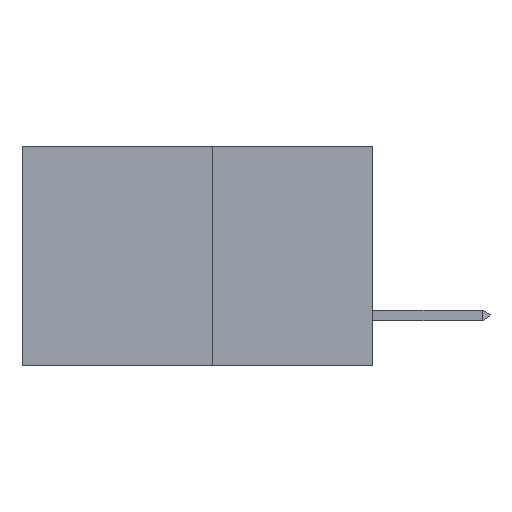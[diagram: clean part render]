
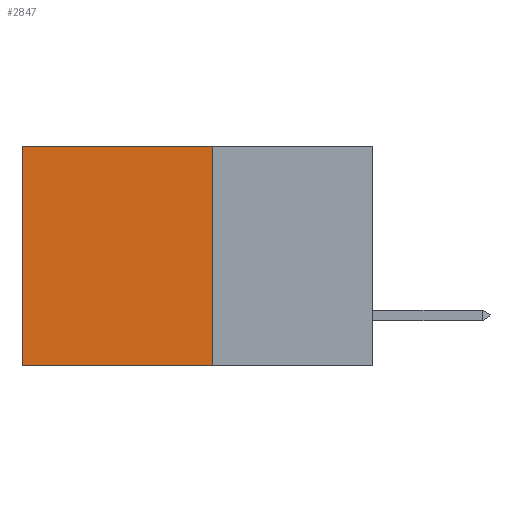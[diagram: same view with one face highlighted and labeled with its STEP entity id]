
A CAD part, left-side view. The second image highlights one B-rep face of the part: STEP entity #2847.
In plain terms, the highlighted planar face has unit normal (-1, 0, 0).
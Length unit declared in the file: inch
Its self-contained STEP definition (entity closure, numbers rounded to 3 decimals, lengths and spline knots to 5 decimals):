
#21 = VERTEX_POINT ( 'NONE', #1891 ) ;
#891 = ORIENTED_EDGE ( 'NONE', *, *, #13866, .F. ) ;
#1246 = ORIENTED_EDGE ( 'NONE', *, *, #14415, .T. ) ;
#1261 = ORIENTED_EDGE ( 'NONE', *, *, #12881, .F. ) ;
#1382 = DIRECTION ( 'NONE',  ( 0., 1., 0. ) ) ;
#1393 = CARTESIAN_POINT ( 'NONE',  ( 0.277, 0.27, -0.37 ) ) ;
#1558 = VERTEX_POINT ( 'NONE', #4974 ) ;
#1891 = CARTESIAN_POINT ( 'NONE',  ( 0.277, 0.27, 0. ) ) ;
#2407 = LINE ( 'NONE', #6162, #14510 ) ;
#2595 = CARTESIAN_POINT ( 'NONE',  ( 0.277, 0.27, -0.37 ) ) ;
#2836 = CARTESIAN_POINT ( 'NONE',  ( 0.277, 0.59, -0.37 ) ) ;
#2847 = ADVANCED_FACE ( 'NONE', ( #6308 ), #4826, .F. ) ;
#3216 = LINE ( 'NONE', #1393, #6069 ) ;
#3367 = CARTESIAN_POINT ( 'NONE',  ( 0.277, 0.59, 0. ) ) ;
#3384 = VECTOR ( 'NONE', #1382, 39.37008 ) ;
#3970 = CARTESIAN_POINT ( 'NONE',  ( 0.277, 0.27, 0. ) ) ;
#3998 = VECTOR ( 'NONE', #5069, 39.37008 ) ;
#4556 = EDGE_CURVE ( 'NONE', #21, #5644, #13021, .T. ) ;
#4626 = DIRECTION ( 'NONE',  ( 1., 0., 0. ) ) ;
#4826 = PLANE ( 'NONE',  #9496 ) ;
#4974 = CARTESIAN_POINT ( 'NONE',  ( 0.277, 0.27, -0.37 ) ) ;
#5069 = DIRECTION ( 'NONE',  ( 0., 1., 0. ) ) ;
#5644 = VERTEX_POINT ( 'NONE', #3367 ) ;
#5672 = ORIENTED_EDGE ( 'NONE', *, *, #4556, .T. ) ;
#6069 = VECTOR ( 'NONE', #11170, 39.37008 ) ;
#6162 = CARTESIAN_POINT ( 'NONE',  ( 0.277, 0.59, -0.37 ) ) ;
#6308 = FACE_OUTER_BOUND ( 'NONE', #12428, .T. ) ;
#9496 = AXIS2_PLACEMENT_3D ( 'NONE', #15103, #4626, #10046 ) ;
#10046 = DIRECTION ( 'NONE',  ( 0., 0., -1. ) ) ;
#10865 = LINE ( 'NONE', #2595, #3998 ) ;
#11058 = DIRECTION ( 'NONE',  ( 0., 0., -1. ) ) ;
#11170 = DIRECTION ( 'NONE',  ( 0., 0., -1. ) ) ;
#11582 = VERTEX_POINT ( 'NONE', #2836 ) ;
#12428 = EDGE_LOOP ( 'NONE', ( #1246, #1261, #891, #5672 ) ) ;
#12881 = EDGE_CURVE ( 'NONE', #1558, #11582, #10865, .T. ) ;
#13021 = LINE ( 'NONE', #3970, #3384 ) ;
#13866 = EDGE_CURVE ( 'NONE', #21, #1558, #3216, .T. ) ;
#14415 = EDGE_CURVE ( 'NONE', #5644, #11582, #2407, .T. ) ;
#14510 = VECTOR ( 'NONE', #11058, 39.37008 ) ;
#15103 = CARTESIAN_POINT ( 'NONE',  ( 0.277, 0.27, -0.37 ) ) ;
